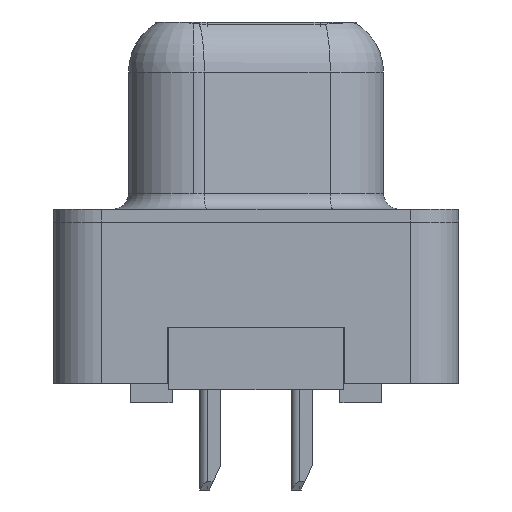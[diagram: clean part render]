
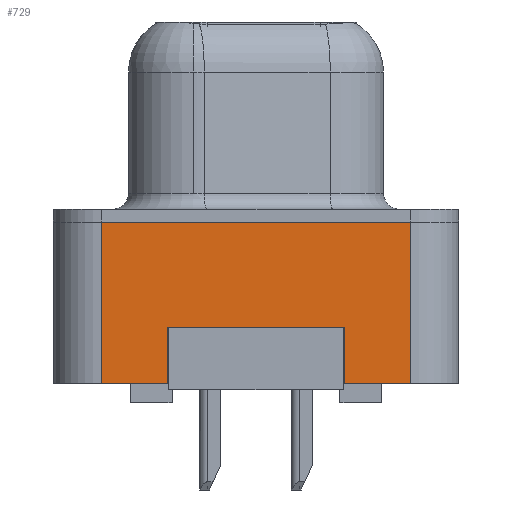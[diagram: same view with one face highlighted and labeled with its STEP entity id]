
A CAD part, left-side view. The second image highlights one B-rep face of the part: STEP entity #729.
In plain terms, the highlighted planar face has unit normal (-1, 0, 0).
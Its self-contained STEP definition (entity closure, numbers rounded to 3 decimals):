
#390 = ORIENTED_EDGE ( 'NONE', *, *, #10018, .T. ) ;
#729 = ADVANCED_FACE ( 'NONE', ( #3267 ), #14329, .T. ) ;
#785 = VECTOR ( 'NONE', #14009, 1000. ) ;
#1033 = VERTEX_POINT ( 'NONE', #4234 ) ;
#1086 = AXIS2_PLACEMENT_3D ( 'NONE', #9368, #2076, #13127 ) ;
#1751 = LINE ( 'NONE', #10405, #785 ) ;
#1862 = LINE ( 'NONE', #3213, #2456 ) ;
#2076 = DIRECTION ( 'NONE',  ( -1., 0., 0. ) ) ;
#2330 = ORIENTED_EDGE ( 'NONE', *, *, #6068, .F. ) ;
#2456 = VECTOR ( 'NONE', #8111, 1000. ) ;
#2640 = LINE ( 'NONE', #11225, #14700 ) ;
#2917 = VECTOR ( 'NONE', #9376, 1000. ) ;
#2941 = VERTEX_POINT ( 'NONE', #6601 ) ;
#2968 = VERTEX_POINT ( 'NONE', #5240 ) ;
#3066 = VERTEX_POINT ( 'NONE', #14369 ) ;
#3140 = VERTEX_POINT ( 'NONE', #8277 ) ;
#3161 = VERTEX_POINT ( 'NONE', #14453 ) ;
#3213 = CARTESIAN_POINT ( 'NONE',  ( -2.905, 2.75, -3.25 ) ) ;
#3267 = FACE_OUTER_BOUND ( 'NONE', #4517, .T. ) ;
#3653 = VECTOR ( 'NONE', #10699, 1000. ) ;
#4234 = CARTESIAN_POINT ( 'NONE',  ( -2.905, -2.75, -5. ) ) ;
#4517 = EDGE_LOOP ( 'NONE', ( #15002, #11675, #12496, #5325, #10506, #390, #8970, #2330 ) ) ;
#4565 = CARTESIAN_POINT ( 'NONE',  ( -2.905, 4.775, -5. ) ) ;
#4673 = DIRECTION ( 'NONE',  ( 0., -1., 0. ) ) ;
#4961 = VECTOR ( 'NONE', #15713, 1000. ) ;
#5240 = CARTESIAN_POINT ( 'NONE',  ( -2.905, 4.775, -5. ) ) ;
#5325 = ORIENTED_EDGE ( 'NONE', *, *, #10113, .F. ) ;
#5885 = LINE ( 'NONE', #6054, #14414 ) ;
#5927 = CARTESIAN_POINT ( 'NONE',  ( -2.905, -4.775, 0. ) ) ;
#6054 = CARTESIAN_POINT ( 'NONE',  ( -2.905, -4.775, -5. ) ) ;
#6068 = EDGE_CURVE ( 'NONE', #2941, #15075, #1862, .T. ) ;
#6489 = EDGE_CURVE ( 'NONE', #2968, #3161, #15559, .T. ) ;
#6601 = CARTESIAN_POINT ( 'NONE',  ( -2.905, -2.75, -3.25 ) ) ;
#6851 = CARTESIAN_POINT ( 'NONE',  ( -2.905, 2.75, -3.25 ) ) ;
#7537 = DIRECTION ( 'NONE',  ( 0., 0., 1. ) ) ;
#7694 = CARTESIAN_POINT ( 'NONE',  ( -2.905, -4.775, 0. ) ) ;
#8111 = DIRECTION ( 'NONE',  ( 0., 1., 0. ) ) ;
#8208 = LINE ( 'NONE', #11980, #3653 ) ;
#8277 = CARTESIAN_POINT ( 'NONE',  ( -2.905, 2.75, -5. ) ) ;
#8362 = CARTESIAN_POINT ( 'NONE',  ( -2.905, -4.775, -5. ) ) ;
#8970 = ORIENTED_EDGE ( 'NONE', *, *, #11528, .F. ) ;
#9368 = CARTESIAN_POINT ( 'NONE',  ( -2.905, -4.775, -5. ) ) ;
#9376 = DIRECTION ( 'NONE',  ( 0., 0., 1. ) ) ;
#9659 = DIRECTION ( 'NONE',  ( 0., -1., 0. ) ) ;
#10018 = EDGE_CURVE ( 'NONE', #2968, #3140, #14448, .T. ) ;
#10113 = EDGE_CURVE ( 'NONE', #3161, #12803, #11783, .T. ) ;
#10405 = CARTESIAN_POINT ( 'NONE',  ( -2.905, -2.75, -3.25 ) ) ;
#10506 = ORIENTED_EDGE ( 'NONE', *, *, #6489, .F. ) ;
#10699 = DIRECTION ( 'NONE',  ( 0., 0., -1. ) ) ;
#11225 = CARTESIAN_POINT ( 'NONE',  ( -2.905, -4.775, -5. ) ) ;
#11528 = EDGE_CURVE ( 'NONE', #15075, #3140, #8208, .T. ) ;
#11675 = ORIENTED_EDGE ( 'NONE', *, *, #15094, .T. ) ;
#11705 = VECTOR ( 'NONE', #4673, 1000. ) ;
#11783 = LINE ( 'NONE', #5927, #4961 ) ;
#11980 = CARTESIAN_POINT ( 'NONE',  ( -2.905, 2.75, -3.25 ) ) ;
#12315 = EDGE_CURVE ( 'NONE', #2941, #1033, #1751, .T. ) ;
#12496 = ORIENTED_EDGE ( 'NONE', *, *, #15470, .T. ) ;
#12803 = VERTEX_POINT ( 'NONE', #7694 ) ;
#13127 = DIRECTION ( 'NONE',  ( 0., 0., 1. ) ) ;
#14009 = DIRECTION ( 'NONE',  ( 0., 0., -1. ) ) ;
#14329 = PLANE ( 'NONE',  #1086 ) ;
#14369 = CARTESIAN_POINT ( 'NONE',  ( -2.905, -4.775, -5. ) ) ;
#14414 = VECTOR ( 'NONE', #9659, 1000. ) ;
#14448 = LINE ( 'NONE', #8362, #11705 ) ;
#14453 = CARTESIAN_POINT ( 'NONE',  ( -2.905, 4.775, 0. ) ) ;
#14700 = VECTOR ( 'NONE', #7537, 1000. ) ;
#15002 = ORIENTED_EDGE ( 'NONE', *, *, #12315, .T. ) ;
#15075 = VERTEX_POINT ( 'NONE', #6851 ) ;
#15094 = EDGE_CURVE ( 'NONE', #1033, #3066, #5885, .T. ) ;
#15470 = EDGE_CURVE ( 'NONE', #3066, #12803, #2640, .T. ) ;
#15559 = LINE ( 'NONE', #4565, #2917 ) ;
#15713 = DIRECTION ( 'NONE',  ( 0., -1., 0. ) ) ;
